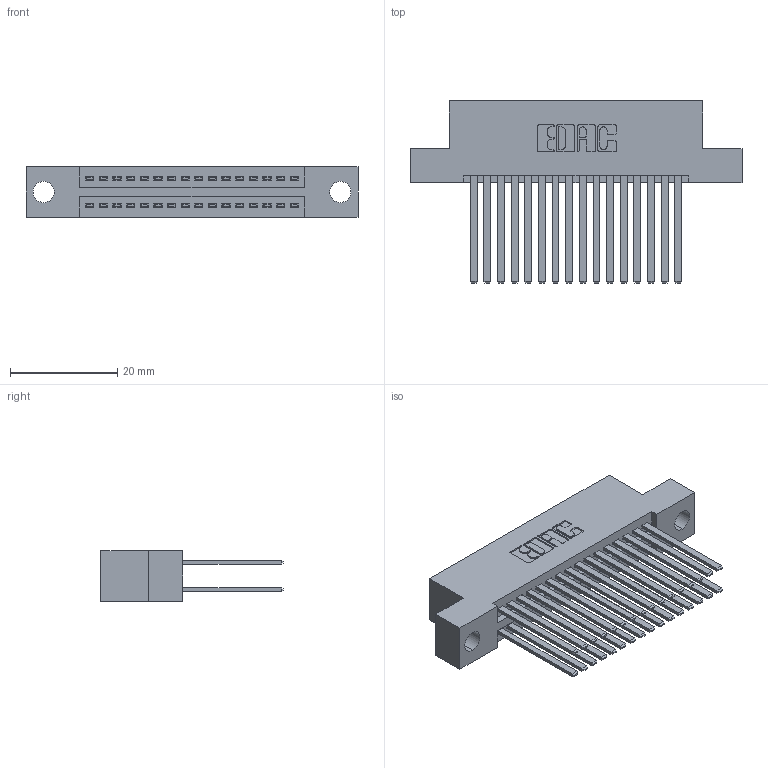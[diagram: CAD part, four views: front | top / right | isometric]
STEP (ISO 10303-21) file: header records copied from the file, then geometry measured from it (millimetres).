
FILE_DESCRIPTION (( 'STEP AP203' ), '1' );
FILE_NAME ('395-032-544-204.STEP', '2021-06-16T20:31:15', ( '' ), ( '' ), 'SwSTEP 2.0', 'SolidWorks 2020', '' );
FILE_SCHEMA (( 'CONFIG_CONTROL_DESIGN' ));
Length unit declared in the file: inch
Products named in the file (3): 345-292-001_345-293-144; 395-032-544-204; 345 Part_Flush Mounting Lugs - 0.156 Dia-TI
Assembly tree (33 placements, depth 2):
  395-032-544-204
    345 Part_Flush Mounting Lugs - 0.156 Dia-TI
    345-292-001_345-293-144  x32
Bounding box: 61.85 x 33.96 x 9.4 mm (x, y, z)
Volume: 6109.4 mm3; surface area: 9693.4 mm2
Topology: 33 solids, 33 shells, 1548 faces, 4569 edges, 3002 vertices
Faces by surface type: plane 1022, cylinder 526
Entity records: 16289 total; most frequent: CARTESIAN_POINT 2758, ORIENTED_EDGE 2690, DIRECTION 2461, EDGE_CURVE 1345, VECTOR 1153, LINE 1153, VERTEX_POINT 894, AXIS2_PLACEMENT_3D 654
